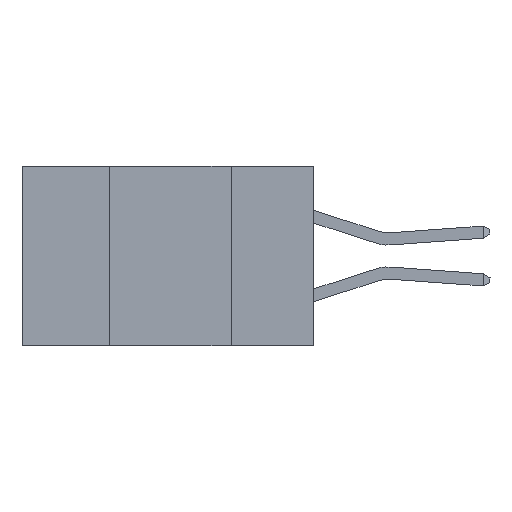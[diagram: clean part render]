
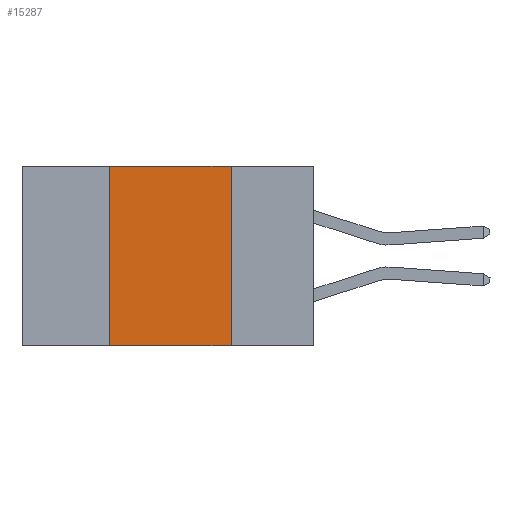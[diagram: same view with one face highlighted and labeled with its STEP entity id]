
A CAD part, left-side view. The second image highlights one B-rep face of the part: STEP entity #15287.
In plain terms, the highlighted planar face has unit normal (-1, 0, 0).
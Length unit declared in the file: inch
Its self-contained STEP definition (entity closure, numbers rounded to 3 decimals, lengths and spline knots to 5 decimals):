
#916 = VECTOR ( 'NONE', #35465, 39.37008 ) ;
#1609 = VECTOR ( 'NONE', #10783, 39.37008 ) ;
#2474 = VERTEX_POINT ( 'NONE', #11814 ) ;
#3169 = VERTEX_POINT ( 'NONE', #24515 ) ;
#4850 = CARTESIAN_POINT ( 'NONE',  ( 0., 0.42, 0. ) ) ;
#9132 = AXIS2_PLACEMENT_3D ( 'NONE', #26567, #39599, #20955 ) ;
#10783 = DIRECTION ( 'NONE',  ( 0., -1., 0. ) ) ;
#10796 = ORIENTED_EDGE ( 'NONE', *, *, #18427, .F. ) ;
#10953 = CARTESIAN_POINT ( 'NONE',  ( 0., 0.6, -0.37 ) ) ;
#11078 = VECTOR ( 'NONE', #34675, 39.37008 ) ;
#11484 = VERTEX_POINT ( 'NONE', #16563 ) ;
#11814 = CARTESIAN_POINT ( 'NONE',  ( 0., 0.17, 0. ) ) ;
#14959 = ORIENTED_EDGE ( 'NONE', *, *, #23750, .F. ) ;
#15287 = ADVANCED_FACE ( 'NONE', ( #25978 ), #20107, .F. ) ;
#16563 = CARTESIAN_POINT ( 'NONE',  ( 0., 0.17, -0.37 ) ) ;
#16941 = EDGE_CURVE ( 'NONE', #2474, #11484, #28632, .T. ) ;
#17064 = DIRECTION ( 'NONE',  ( 0., -1., 0. ) ) ;
#17312 = CARTESIAN_POINT ( 'NONE',  ( 0., 0.6, 0. ) ) ;
#18427 = EDGE_CURVE ( 'NONE', #22781, #3169, #31491, .T. ) ;
#19094 = CARTESIAN_POINT ( 'NONE',  ( 0., 0.17, 0. ) ) ;
#19318 = ORIENTED_EDGE ( 'NONE', *, *, #36822, .T. ) ;
#20107 = PLANE ( 'NONE',  #9132 ) ;
#20955 = DIRECTION ( 'NONE',  ( 0., 0., -1. ) ) ;
#22073 = LINE ( 'NONE', #10953, #23088 ) ;
#22179 = EDGE_LOOP ( 'NONE', ( #40006, #14959, #10796, #19318 ) ) ;
#22781 = VERTEX_POINT ( 'NONE', #34652 ) ;
#23088 = VECTOR ( 'NONE', #17064, 39.37008 ) ;
#23750 = EDGE_CURVE ( 'NONE', #3169, #2474, #25715, .T. ) ;
#24515 = CARTESIAN_POINT ( 'NONE',  ( 0., 0.42, 0. ) ) ;
#25715 = LINE ( 'NONE', #17312, #1609 ) ;
#25978 = FACE_OUTER_BOUND ( 'NONE', #22179, .T. ) ;
#26567 = CARTESIAN_POINT ( 'NONE',  ( 0., 0.6, 0. ) ) ;
#28632 = LINE ( 'NONE', #19094, #11078 ) ;
#31491 = LINE ( 'NONE', #4850, #916 ) ;
#34652 = CARTESIAN_POINT ( 'NONE',  ( 0., 0.42, -0.37 ) ) ;
#34675 = DIRECTION ( 'NONE',  ( 0., 0., -1. ) ) ;
#35465 = DIRECTION ( 'NONE',  ( 0., 0., 1. ) ) ;
#36822 = EDGE_CURVE ( 'NONE', #22781, #11484, #22073, .T. ) ;
#39599 = DIRECTION ( 'NONE',  ( 1., 0., 0. ) ) ;
#40006 = ORIENTED_EDGE ( 'NONE', *, *, #16941, .F. ) ;
